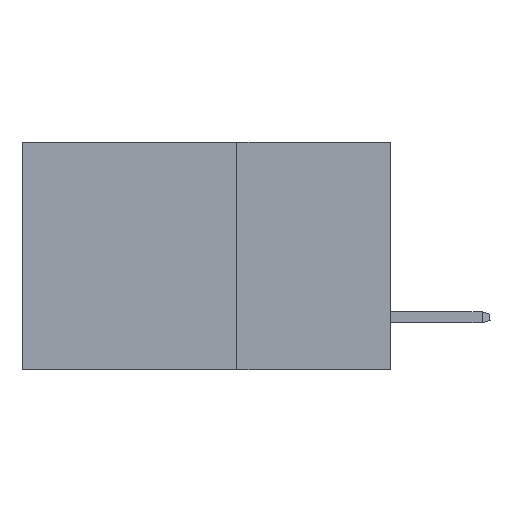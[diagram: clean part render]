
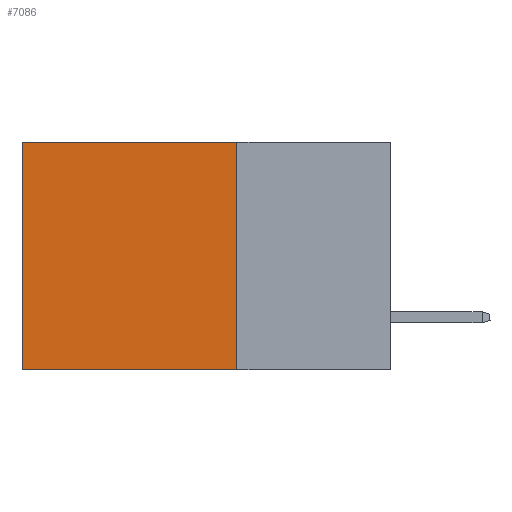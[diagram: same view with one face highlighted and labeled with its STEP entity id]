
A CAD part, left-side view. The second image highlights one B-rep face of the part: STEP entity #7086.
In plain terms, the highlighted planar face has unit normal (-1, 0, 0).
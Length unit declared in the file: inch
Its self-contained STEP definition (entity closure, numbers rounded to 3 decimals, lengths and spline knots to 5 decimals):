
#1204 = CARTESIAN_POINT ( 'NONE',  ( 0.2875, 0.25, 0. ) ) ;
#1771 = LINE ( 'NONE', #1204, #8465 ) ;
#1904 = VERTEX_POINT ( 'NONE', #12906 ) ;
#2244 = ORIENTED_EDGE ( 'NONE', *, *, #3377, .T. ) ;
#3302 = EDGE_LOOP ( 'NONE', ( #2244, #8831, #12378, #15210 ) ) ;
#3377 = EDGE_CURVE ( 'NONE', #1904, #3904, #13045, .T. ) ;
#3598 = CARTESIAN_POINT ( 'NONE',  ( 0.2875, 0.6, -0.37 ) ) ;
#3645 = VECTOR ( 'NONE', #7522, 39.37008 ) ;
#3904 = VERTEX_POINT ( 'NONE', #3598 ) ;
#3990 = CARTESIAN_POINT ( 'NONE',  ( 0.2875, 0.25, 0. ) ) ;
#5222 = CARTESIAN_POINT ( 'NONE',  ( 0.2875, 0.25, 0. ) ) ;
#5288 = AXIS2_PLACEMENT_3D ( 'NONE', #3990, #5432, #15169 ) ;
#5432 = DIRECTION ( 'NONE',  ( 1., 0., 0. ) ) ;
#6261 = EDGE_CURVE ( 'NONE', #17090, #3904, #9268, .T. ) ;
#6442 = DIRECTION ( 'NONE',  ( 0., 0., -1. ) ) ;
#6588 = CARTESIAN_POINT ( 'NONE',  ( 0.2875, 0.6, 0. ) ) ;
#7086 = ADVANCED_FACE ( 'NONE', ( #10301 ), #15114, .F. ) ;
#7522 = DIRECTION ( 'NONE',  ( 0., 0., -1. ) ) ;
#8315 = LINE ( 'NONE', #10309, #3645 ) ;
#8465 = VECTOR ( 'NONE', #13880, 39.37008 ) ;
#8831 = ORIENTED_EDGE ( 'NONE', *, *, #6261, .F. ) ;
#9120 = DIRECTION ( 'NONE',  ( 0., 1., 0. ) ) ;
#9235 = VERTEX_POINT ( 'NONE', #5222 ) ;
#9268 = LINE ( 'NONE', #14597, #16129 ) ;
#9353 = CARTESIAN_POINT ( 'NONE',  ( 0.2875, 0.25, -0.37 ) ) ;
#9377 = EDGE_CURVE ( 'NONE', #9235, #1904, #1771, .T. ) ;
#9769 = VECTOR ( 'NONE', #6442, 39.37008 ) ;
#10301 = FACE_OUTER_BOUND ( 'NONE', #3302, .T. ) ;
#10309 = CARTESIAN_POINT ( 'NONE',  ( 0.2875, 0.25, 0. ) ) ;
#12378 = ORIENTED_EDGE ( 'NONE', *, *, #17545, .F. ) ;
#12906 = CARTESIAN_POINT ( 'NONE',  ( 0.2875, 0.6, 0. ) ) ;
#13045 = LINE ( 'NONE', #6588, #9769 ) ;
#13880 = DIRECTION ( 'NONE',  ( 0., 1., 0. ) ) ;
#14597 = CARTESIAN_POINT ( 'NONE',  ( 0.2875, 0.25, -0.37 ) ) ;
#15114 = PLANE ( 'NONE',  #5288 ) ;
#15169 = DIRECTION ( 'NONE',  ( 0., 0., -1. ) ) ;
#15210 = ORIENTED_EDGE ( 'NONE', *, *, #9377, .T. ) ;
#16129 = VECTOR ( 'NONE', #9120, 39.37008 ) ;
#17090 = VERTEX_POINT ( 'NONE', #9353 ) ;
#17545 = EDGE_CURVE ( 'NONE', #9235, #17090, #8315, .T. ) ;
